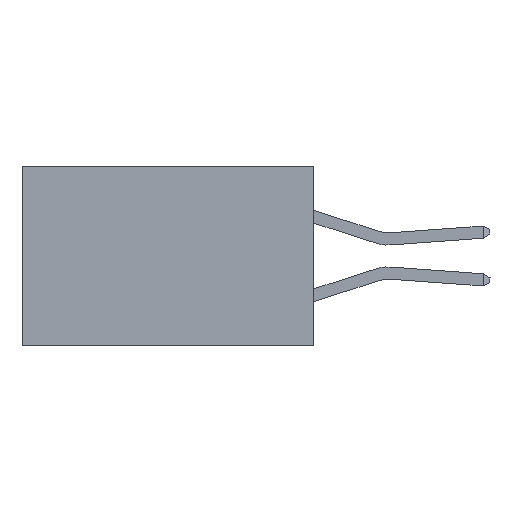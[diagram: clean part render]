
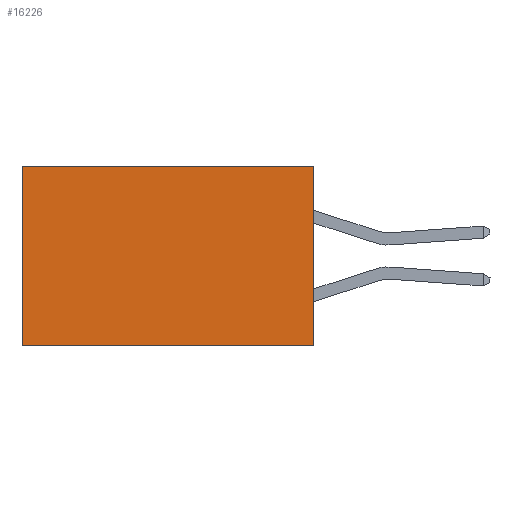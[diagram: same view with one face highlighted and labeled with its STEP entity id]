
A CAD part, left-side view. The second image highlights one B-rep face of the part: STEP entity #16226.
In plain terms, the highlighted planar face has unit normal (-1, 0, 0).
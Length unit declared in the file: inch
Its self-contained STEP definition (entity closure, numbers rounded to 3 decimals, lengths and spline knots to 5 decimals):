
#76 = CARTESIAN_POINT ( 'NONE',  ( 0.2875, 0., 0. ) ) ;
#213 = LINE ( 'NONE', #21558, #4844 ) ;
#412 = VERTEX_POINT ( 'NONE', #21924 ) ;
#1753 = DIRECTION ( 'NONE',  ( 0., 1., 0. ) ) ;
#4844 = VECTOR ( 'NONE', #9705, 39.37008 ) ;
#5788 = DIRECTION ( 'NONE',  ( 0., 0., -1. ) ) ;
#5993 = CARTESIAN_POINT ( 'NONE',  ( 0.2875, 0.6, -0.37 ) ) ;
#6973 = VERTEX_POINT ( 'NONE', #22096 ) ;
#7391 = VECTOR ( 'NONE', #1753, 39.37008 ) ;
#7945 = ORIENTED_EDGE ( 'NONE', *, *, #9221, .T. ) ;
#8245 = EDGE_CURVE ( 'NONE', #412, #13765, #12897, .T. ) ;
#9221 = EDGE_CURVE ( 'NONE', #6973, #18958, #213, .T. ) ;
#9705 = DIRECTION ( 'NONE',  ( 0., 1., 0. ) ) ;
#9931 = PLANE ( 'NONE',  #15232 ) ;
#10100 = DIRECTION ( 'NONE',  ( 0., 0., -1. ) ) ;
#10523 = DIRECTION ( 'NONE',  ( 0., 0., -1. ) ) ;
#11891 = DIRECTION ( 'NONE',  ( 1., 0., 0. ) ) ;
#12897 = LINE ( 'NONE', #19463, #7391 ) ;
#13765 = VERTEX_POINT ( 'NONE', #5993 ) ;
#14706 = EDGE_CURVE ( 'NONE', #6973, #412, #16407, .T. ) ;
#14776 = FACE_OUTER_BOUND ( 'NONE', #16101, .T. ) ;
#15232 = AXIS2_PLACEMENT_3D ( 'NONE', #76, #11891, #10100 ) ;
#16101 = EDGE_LOOP ( 'NONE', ( #17882, #20655, #21846, #7945 ) ) ;
#16226 = ADVANCED_FACE ( 'NONE', ( #14776 ), #9931, .F. ) ;
#16407 = LINE ( 'NONE', #25329, #18875 ) ;
#17164 = EDGE_CURVE ( 'NONE', #18958, #13765, #22786, .T. ) ;
#17882 = ORIENTED_EDGE ( 'NONE', *, *, #17164, .T. ) ;
#18295 = CARTESIAN_POINT ( 'NONE',  ( 0.2875, 0.6, 0. ) ) ;
#18875 = VECTOR ( 'NONE', #5788, 39.37008 ) ;
#18958 = VERTEX_POINT ( 'NONE', #23767 ) ;
#19463 = CARTESIAN_POINT ( 'NONE',  ( 0.2875, 0., -0.37 ) ) ;
#20655 = ORIENTED_EDGE ( 'NONE', *, *, #8245, .F. ) ;
#21558 = CARTESIAN_POINT ( 'NONE',  ( 0.2875, 0., 0. ) ) ;
#21846 = ORIENTED_EDGE ( 'NONE', *, *, #14706, .F. ) ;
#21867 = VECTOR ( 'NONE', #10523, 39.37008 ) ;
#21924 = CARTESIAN_POINT ( 'NONE',  ( 0.2875, 0., -0.37 ) ) ;
#22096 = CARTESIAN_POINT ( 'NONE',  ( 0.2875, 0., 0. ) ) ;
#22786 = LINE ( 'NONE', #18295, #21867 ) ;
#23767 = CARTESIAN_POINT ( 'NONE',  ( 0.2875, 0.6, 0. ) ) ;
#25329 = CARTESIAN_POINT ( 'NONE',  ( 0.2875, 0., 0. ) ) ;
